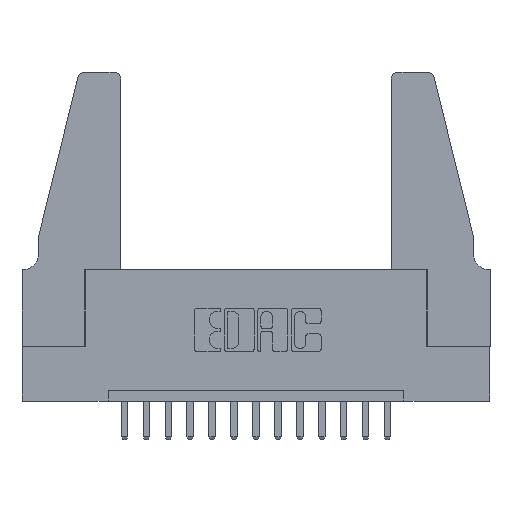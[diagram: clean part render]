
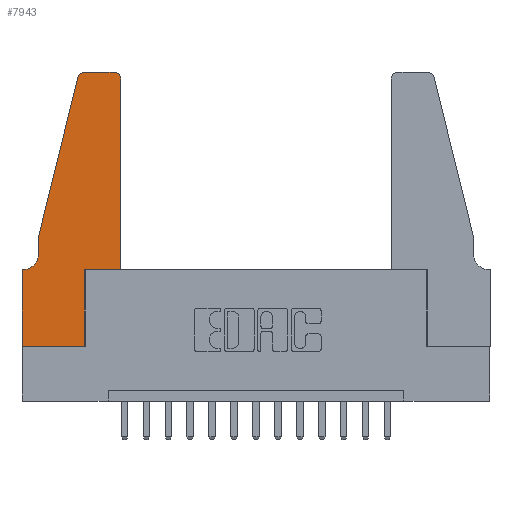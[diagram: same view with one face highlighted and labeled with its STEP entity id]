
A CAD part, top view. The second image highlights one B-rep face of the part: STEP entity #7943.
In plain terms, the highlighted planar face has unit normal (0, 0, 1).
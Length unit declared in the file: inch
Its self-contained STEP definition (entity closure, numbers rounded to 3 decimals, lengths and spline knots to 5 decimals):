
#356 = LINE ( 'NONE', #7973, #1147 ) ;
#507 = AXIS2_PLACEMENT_3D ( 'NONE', #2089, #11868, #11709 ) ;
#698 = DIRECTION ( 'NONE',  ( 1., 0., 0. ) ) ;
#714 = CARTESIAN_POINT ( 'NONE',  ( 0.0055, 0.35, 0.37 ) ) ;
#775 = EDGE_CURVE ( 'NONE', #5898, #2322, #8133, .T. ) ;
#790 = LINE ( 'NONE', #14245, #10372 ) ;
#918 = CARTESIAN_POINT ( 'NONE',  ( 0., 0., 0.37 ) ) ;
#1147 = VECTOR ( 'NONE', #14361, 39.37008 ) ;
#1395 = LINE ( 'NONE', #13972, #8853 ) ;
#2053 = VECTOR ( 'NONE', #4607, 39.37008 ) ;
#2065 = CIRCLE ( 'NONE', #507, 0.07 ) ;
#2089 = CARTESIAN_POINT ( 'NONE',  ( 0.0055, 0.42, 0.37 ) ) ;
#2097 = VERTEX_POINT ( 'NONE', #7566 ) ;
#2118 = VERTEX_POINT ( 'NONE', #3859 ) ;
#2193 = CARTESIAN_POINT ( 'NONE',  ( 0.2605, 1.25, 0.37 ) ) ;
#2322 = VERTEX_POINT ( 'NONE', #15884 ) ;
#2450 = CARTESIAN_POINT ( 'NONE',  ( 0.2865, 0., 0.37 ) ) ;
#2478 = VECTOR ( 'NONE', #6886, 39.37008 ) ;
#2647 = AXIS2_PLACEMENT_3D ( 'NONE', #11925, #14365, #11770 ) ;
#2814 = ORIENTED_EDGE ( 'NONE', *, *, #14910, .T. ) ;
#3011 = LINE ( 'NONE', #15227, #7551 ) ;
#3177 = DIRECTION ( 'NONE',  ( 1., 0., 0. ) ) ;
#3288 = DIRECTION ( 'NONE',  ( 0., 0., 1. ) ) ;
#3536 = EDGE_CURVE ( 'NONE', #5322, #5898, #5087, .T. ) ;
#3593 = EDGE_CURVE ( 'NONE', #15015, #10371, #5184, .T. ) ;
#3850 = FACE_OUTER_BOUND ( 'NONE', #11544, .T. ) ;
#3859 = CARTESIAN_POINT ( 'NONE',  ( 0., 0., 0.37 ) ) ;
#4166 = LINE ( 'NONE', #10518, #2478 ) ;
#4347 = DIRECTION ( 'NONE',  ( -0.239, -0.971, 0. ) ) ;
#4607 = DIRECTION ( 'NONE',  ( -1., 0., 0. ) ) ;
#4870 = CARTESIAN_POINT ( 'NONE',  ( 0.0755, 0.5, 0.37 ) ) ;
#5087 = CIRCLE ( 'NONE', #14500, 0.03 ) ;
#5184 = LINE ( 'NONE', #5812, #7461 ) ;
#5296 = ORIENTED_EDGE ( 'NONE', *, *, #11476, .T. ) ;
#5322 = VERTEX_POINT ( 'NONE', #14506 ) ;
#5444 = CARTESIAN_POINT ( 'NONE',  ( 0.0755, 0.5, 0.37 ) ) ;
#5702 = DIRECTION ( 'NONE',  ( 0., 0., 1. ) ) ;
#5812 = CARTESIAN_POINT ( 'NONE',  ( 0.2865, 0.35, 0.37 ) ) ;
#5898 = VERTEX_POINT ( 'NONE', #7821 ) ;
#6826 = CARTESIAN_POINT ( 'NONE',  ( 0.4205, 1.22, 0.37 ) ) ;
#6886 = DIRECTION ( 'NONE',  ( -1., 0., 0. ) ) ;
#7004 = ORIENTED_EDGE ( 'NONE', *, *, #14660, .T. ) ;
#7304 = EDGE_CURVE ( 'NONE', #14010, #14323, #4166, .T. ) ;
#7385 = ORIENTED_EDGE ( 'NONE', *, *, #3536, .T. ) ;
#7386 = ORIENTED_EDGE ( 'NONE', *, *, #14657, .T. ) ;
#7461 = VECTOR ( 'NONE', #15876, 39.37008 ) ;
#7551 = VECTOR ( 'NONE', #11568, 39.37008 ) ;
#7566 = CARTESIAN_POINT ( 'NONE',  ( 0.4505, 0.35, 0.37 ) ) ;
#7821 = CARTESIAN_POINT ( 'NONE',  ( 0.4205, 1.25, 0.37 ) ) ;
#7943 = ADVANCED_FACE ( 'NONE', ( #3850 ), #9299, .T. ) ;
#7973 = CARTESIAN_POINT ( 'NONE',  ( 0.4505, 0.35, 0.37 ) ) ;
#8133 = LINE ( 'NONE', #2193, #2053 ) ;
#8384 = VERTEX_POINT ( 'NONE', #10203 ) ;
#8853 = VECTOR ( 'NONE', #11854, 39.37008 ) ;
#9023 = EDGE_CURVE ( 'NONE', #10371, #2097, #1395, .T. ) ;
#9299 = PLANE ( 'NONE',  #11863 ) ;
#9342 = CARTESIAN_POINT ( 'NONE',  ( 0., 0.35, 0.37 ) ) ;
#9778 = DIRECTION ( 'NONE',  ( 0., -1., 0. ) ) ;
#10112 = CIRCLE ( 'NONE', #2647, 0.03 ) ;
#10172 = ORIENTED_EDGE ( 'NONE', *, *, #775, .T. ) ;
#10203 = CARTESIAN_POINT ( 'NONE',  ( 0.0755, 0.42, 0.37 ) ) ;
#10371 = VERTEX_POINT ( 'NONE', #15736 ) ;
#10372 = VECTOR ( 'NONE', #4347, 39.37008 ) ;
#10434 = ORIENTED_EDGE ( 'NONE', *, *, #9023, .T. ) ;
#10518 = CARTESIAN_POINT ( 'NONE',  ( 0.0755, 0.35, 0.37 ) ) ;
#10598 = ORIENTED_EDGE ( 'NONE', *, *, #11462, .T. ) ;
#10708 = LINE ( 'NONE', #4870, #14034 ) ;
#11462 = EDGE_CURVE ( 'NONE', #11889, #14503, #790, .T. ) ;
#11476 = EDGE_CURVE ( 'NONE', #2097, #5322, #356, .T. ) ;
#11544 = EDGE_LOOP ( 'NONE', ( #10172, #15649, #10598, #2814, #7386, #12532, #15968, #7004, #15037, #10434, #5296, #7385 ) ) ;
#11568 = DIRECTION ( 'NONE',  ( 0., -1., 0. ) ) ;
#11709 = DIRECTION ( 'NONE',  ( -1., 0., 0. ) ) ;
#11770 = DIRECTION ( 'NONE',  ( 1., 0., 0. ) ) ;
#11854 = DIRECTION ( 'NONE',  ( 1., 0., 0. ) ) ;
#11863 = AXIS2_PLACEMENT_3D ( 'NONE', #9342, #3288, #3177 ) ;
#11868 = DIRECTION ( 'NONE',  ( 0., 0., -1. ) ) ;
#11889 = VERTEX_POINT ( 'NONE', #12479 ) ;
#11925 = CARTESIAN_POINT ( 'NONE',  ( 0.284, 1.22, 0.37 ) ) ;
#12479 = CARTESIAN_POINT ( 'NONE',  ( 0.25487, 1.22718, 0.37 ) ) ;
#12532 = ORIENTED_EDGE ( 'NONE', *, *, #7304, .T. ) ;
#13023 = VECTOR ( 'NONE', #698, 39.37008 ) ;
#13697 = CARTESIAN_POINT ( 'NONE',  ( 0., 0.35, 0.37 ) ) ;
#13972 = CARTESIAN_POINT ( 'NONE',  ( 0.4505, 0.35, 0.37 ) ) ;
#14010 = VERTEX_POINT ( 'NONE', #714 ) ;
#14034 = VECTOR ( 'NONE', #9778, 39.37008 ) ;
#14245 = CARTESIAN_POINT ( 'NONE',  ( 0.0755, 0.5, 0.37 ) ) ;
#14323 = VERTEX_POINT ( 'NONE', #13697 ) ;
#14361 = DIRECTION ( 'NONE',  ( 0., 1., 0. ) ) ;
#14365 = DIRECTION ( 'NONE',  ( 0., 0., 1. ) ) ;
#14442 = EDGE_CURVE ( 'NONE', #14323, #2118, #3011, .T. ) ;
#14500 = AXIS2_PLACEMENT_3D ( 'NONE', #6826, #5702, #15699 ) ;
#14503 = VERTEX_POINT ( 'NONE', #5444 ) ;
#14506 = CARTESIAN_POINT ( 'NONE',  ( 0.4505, 1.22, 0.37 ) ) ;
#14642 = EDGE_CURVE ( 'NONE', #2322, #11889, #10112, .T. ) ;
#14657 = EDGE_CURVE ( 'NONE', #8384, #14010, #2065, .T. ) ;
#14660 = EDGE_CURVE ( 'NONE', #2118, #15015, #14829, .T. ) ;
#14829 = LINE ( 'NONE', #918, #13023 ) ;
#14910 = EDGE_CURVE ( 'NONE', #14503, #8384, #10708, .T. ) ;
#15015 = VERTEX_POINT ( 'NONE', #2450 ) ;
#15037 = ORIENTED_EDGE ( 'NONE', *, *, #3593, .T. ) ;
#15227 = CARTESIAN_POINT ( 'NONE',  ( 0., 0., 0.37 ) ) ;
#15649 = ORIENTED_EDGE ( 'NONE', *, *, #14642, .T. ) ;
#15699 = DIRECTION ( 'NONE',  ( 1., 0., 0. ) ) ;
#15736 = CARTESIAN_POINT ( 'NONE',  ( 0.2865, 0.35, 0.37 ) ) ;
#15876 = DIRECTION ( 'NONE',  ( 0., 1., 0. ) ) ;
#15884 = CARTESIAN_POINT ( 'NONE',  ( 0.284, 1.25, 0.37 ) ) ;
#15968 = ORIENTED_EDGE ( 'NONE', *, *, #14442, .T. ) ;
